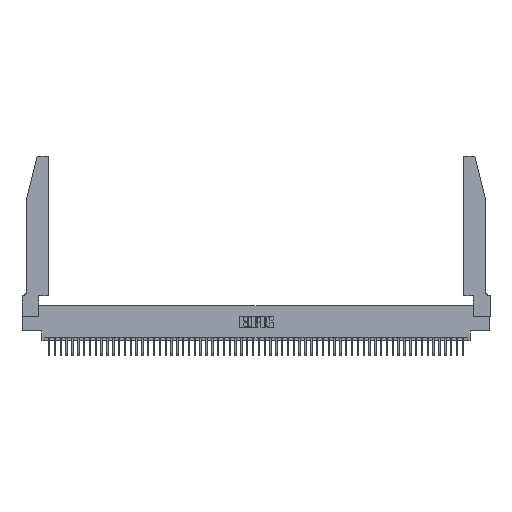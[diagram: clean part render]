
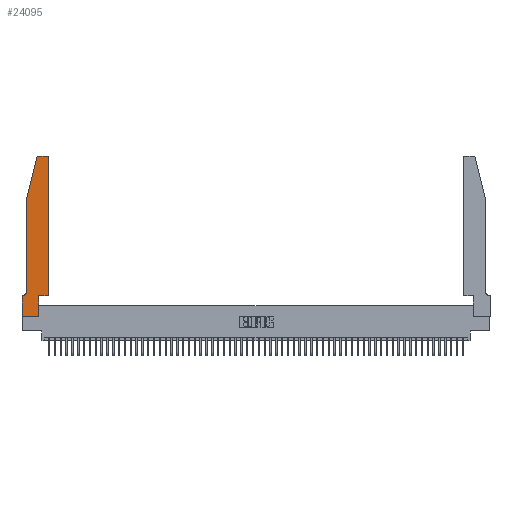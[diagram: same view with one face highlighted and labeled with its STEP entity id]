
A CAD part, top view. The second image highlights one B-rep face of the part: STEP entity #24095.
In plain terms, the highlighted planar face has unit normal (0, 0, 1).
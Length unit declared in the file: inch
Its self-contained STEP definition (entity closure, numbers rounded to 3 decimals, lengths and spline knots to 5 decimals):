
#337 = AXIS2_PLACEMENT_3D ( 'NONE', #19456, #49234, #23762 ) ;
#1120 = CARTESIAN_POINT ( 'NONE',  ( 0.4205, 2.75, 0.37 ) ) ;
#1465 = CARTESIAN_POINT ( 'NONE',  ( 0., 0., 0.37 ) ) ;
#1856 = AXIS2_PLACEMENT_3D ( 'NONE', #42576, #17095, #46843 ) ;
#1922 = AXIS2_PLACEMENT_3D ( 'NONE', #6892, #36635, #11171 ) ;
#1955 = EDGE_CURVE ( 'NONE', #13772, #27089, #21407, .T. ) ;
#2483 = AXIS2_PLACEMENT_3D ( 'NONE', #31450, #44285, #18793 ) ;
#2968 = DIRECTION ( 'NONE',  ( 0., -1., 0. ) ) ;
#3579 = CARTESIAN_POINT ( 'NONE',  ( 0., 0., 0.37 ) ) ;
#4374 = LINE ( 'NONE', #47335, #25653 ) ;
#4497 = CARTESIAN_POINT ( 'NONE',  ( 0.4505, 0.35, 0.37 ) ) ;
#4533 = LINE ( 'NONE', #18354, #25802 ) ;
#4956 = DIRECTION ( 'NONE',  ( 0., -1., 0. ) ) ;
#5201 = VECTOR ( 'NONE', #12156, 39.37008 ) ;
#5822 = CARTESIAN_POINT ( 'NONE',  ( 0.0755, 2., 0.37 ) ) ;
#6557 = LINE ( 'NONE', #3579, #5201 ) ;
#6892 = CARTESIAN_POINT ( 'NONE',  ( 0.0055, 0.42, 0.37 ) ) ;
#7888 = CIRCLE ( 'NONE', #337, 0.03 ) ;
#9234 = VERTEX_POINT ( 'NONE', #1120 ) ;
#11082 = VECTOR ( 'NONE', #4956, 39.37008 ) ;
#11171 = DIRECTION ( 'NONE',  ( -1., 0., 0. ) ) ;
#11307 = FACE_OUTER_BOUND ( 'NONE', #47465, .T. ) ;
#11352 = EDGE_CURVE ( 'NONE', #9234, #47479, #4374, .T. ) ;
#11476 = VECTOR ( 'NONE', #53965, 39.37008 ) ;
#11644 = CARTESIAN_POINT ( 'NONE',  ( 0.2865, 0.35, 0.37 ) ) ;
#11789 = VECTOR ( 'NONE', #41474, 39.37008 ) ;
#12156 = DIRECTION ( 'NONE',  ( 1., 0., 0. ) ) ;
#12590 = EDGE_CURVE ( 'NONE', #44897, #9234, #29508, .T. ) ;
#13052 = DIRECTION ( 'NONE',  ( 1., 0., 0. ) ) ;
#13772 = VERTEX_POINT ( 'NONE', #37748 ) ;
#14121 = EDGE_CURVE ( 'NONE', #33669, #23694, #28674, .T. ) ;
#15926 = ORIENTED_EDGE ( 'NONE', *, *, #1955, .T. ) ;
#16284 = EDGE_CURVE ( 'NONE', #50764, #33669, #6557, .T. ) ;
#17095 = DIRECTION ( 'NONE',  ( 0., 0., 1. ) ) ;
#17925 = CARTESIAN_POINT ( 'NONE',  ( 0., 0., 0.37 ) ) ;
#18354 = CARTESIAN_POINT ( 'NONE',  ( 0.4505, 0.35, 0.37 ) ) ;
#18793 = DIRECTION ( 'NONE',  ( 1., 0., 0. ) ) ;
#19456 = CARTESIAN_POINT ( 'NONE',  ( 0.284, 2.72, 0.37 ) ) ;
#21407 = LINE ( 'NONE', #37072, #11476 ) ;
#22044 = ORIENTED_EDGE ( 'NONE', *, *, #38626, .T. ) ;
#22248 = LINE ( 'NONE', #4497, #43533 ) ;
#23079 = LINE ( 'NONE', #37208, #11789 ) ;
#23194 = ORIENTED_EDGE ( 'NONE', *, *, #24812, .T. ) ;
#23694 = VERTEX_POINT ( 'NONE', #11644 ) ;
#23709 = LINE ( 'NONE', #17925, #11082 ) ;
#23762 = DIRECTION ( 'NONE',  ( 1., 0., 0. ) ) ;
#23833 = CARTESIAN_POINT ( 'NONE',  ( 0.4505, 0.35, 0.37 ) ) ;
#24095 = ADVANCED_FACE ( 'NONE', ( #11307 ), #40015, .T. ) ;
#24812 = EDGE_CURVE ( 'NONE', #47479, #26191, #7888, .T. ) ;
#25615 = EDGE_CURVE ( 'NONE', #26191, #43483, #23079, .T. ) ;
#25653 = VECTOR ( 'NONE', #43073, 39.37008 ) ;
#25802 = VECTOR ( 'NONE', #44057, 39.37008 ) ;
#26191 = VERTEX_POINT ( 'NONE', #28221 ) ;
#26787 = VERTEX_POINT ( 'NONE', #41174 ) ;
#27089 = VERTEX_POINT ( 'NONE', #39281 ) ;
#27273 = ORIENTED_EDGE ( 'NONE', *, *, #16284, .T. ) ;
#28084 = ORIENTED_EDGE ( 'NONE', *, *, #36572, .T. ) ;
#28221 = CARTESIAN_POINT ( 'NONE',  ( 0.25487, 2.72718, 0.37 ) ) ;
#28674 = LINE ( 'NONE', #31579, #41311 ) ;
#29508 = CIRCLE ( 'NONE', #1856, 0.03 ) ;
#30408 = CIRCLE ( 'NONE', #1922, 0.07 ) ;
#30502 = ORIENTED_EDGE ( 'NONE', *, *, #11352, .T. ) ;
#31216 = ORIENTED_EDGE ( 'NONE', *, *, #40775, .T. ) ;
#31450 = CARTESIAN_POINT ( 'NONE',  ( 0., 0.35, 0.37 ) ) ;
#31579 = CARTESIAN_POINT ( 'NONE',  ( 0.2865, 0.35, 0.37 ) ) ;
#31886 = ORIENTED_EDGE ( 'NONE', *, *, #25615, .T. ) ;
#32110 = VERTEX_POINT ( 'NONE', #23833 ) ;
#32732 = CARTESIAN_POINT ( 'NONE',  ( 0.0755, 2., 0.37 ) ) ;
#33669 = VERTEX_POINT ( 'NONE', #50611 ) ;
#35872 = DIRECTION ( 'NONE',  ( 0., 1., 0. ) ) ;
#36572 = EDGE_CURVE ( 'NONE', #32110, #44897, #4533, .T. ) ;
#36635 = DIRECTION ( 'NONE',  ( 0., 0., -1. ) ) ;
#36973 = CARTESIAN_POINT ( 'NONE',  ( 0.284, 2.75, 0.37 ) ) ;
#37072 = CARTESIAN_POINT ( 'NONE',  ( 0.0755, 0.35, 0.37 ) ) ;
#37187 = EDGE_CURVE ( 'NONE', #26787, #13772, #30408, .T. ) ;
#37208 = CARTESIAN_POINT ( 'NONE',  ( 0.0755, 2., 0.37 ) ) ;
#37517 = VECTOR ( 'NONE', #2968, 39.37008 ) ;
#37748 = CARTESIAN_POINT ( 'NONE',  ( 0.0055, 0.35, 0.37 ) ) ;
#38626 = EDGE_CURVE ( 'NONE', #23694, #32110, #22248, .T. ) ;
#38958 = EDGE_CURVE ( 'NONE', #43483, #26787, #50160, .T. ) ;
#39281 = CARTESIAN_POINT ( 'NONE',  ( 0., 0.35, 0.37 ) ) ;
#40015 = PLANE ( 'NONE',  #2483 ) ;
#40775 = EDGE_CURVE ( 'NONE', #27089, #50764, #23709, .T. ) ;
#41174 = CARTESIAN_POINT ( 'NONE',  ( 0.0755, 0.42, 0.37 ) ) ;
#41311 = VECTOR ( 'NONE', #35872, 39.37008 ) ;
#41474 = DIRECTION ( 'NONE',  ( -0.239, -0.971, 0. ) ) ;
#42576 = CARTESIAN_POINT ( 'NONE',  ( 0.4205, 2.72, 0.37 ) ) ;
#43073 = DIRECTION ( 'NONE',  ( -1., 0., 0. ) ) ;
#43483 = VERTEX_POINT ( 'NONE', #5822 ) ;
#43533 = VECTOR ( 'NONE', #13052, 39.37008 ) ;
#44057 = DIRECTION ( 'NONE',  ( 0., 1., 0. ) ) ;
#44285 = DIRECTION ( 'NONE',  ( 0., 0., 1. ) ) ;
#44897 = VERTEX_POINT ( 'NONE', #54198 ) ;
#46729 = ORIENTED_EDGE ( 'NONE', *, *, #12590, .T. ) ;
#46843 = DIRECTION ( 'NONE',  ( 1., 0., 0. ) ) ;
#47263 = ORIENTED_EDGE ( 'NONE', *, *, #14121, .T. ) ;
#47335 = CARTESIAN_POINT ( 'NONE',  ( 0.2605, 2.75, 0.37 ) ) ;
#47465 = EDGE_LOOP ( 'NONE', ( #30502, #23194, #31886, #47915, #52448, #15926, #31216, #27273, #47263, #22044, #28084, #46729 ) ) ;
#47479 = VERTEX_POINT ( 'NONE', #36973 ) ;
#47915 = ORIENTED_EDGE ( 'NONE', *, *, #38958, .T. ) ;
#49234 = DIRECTION ( 'NONE',  ( 0., 0., 1. ) ) ;
#50160 = LINE ( 'NONE', #32732, #37517 ) ;
#50611 = CARTESIAN_POINT ( 'NONE',  ( 0.2865, 0., 0.37 ) ) ;
#50764 = VERTEX_POINT ( 'NONE', #1465 ) ;
#52448 = ORIENTED_EDGE ( 'NONE', *, *, #37187, .T. ) ;
#53965 = DIRECTION ( 'NONE',  ( -1., 0., 0. ) ) ;
#54198 = CARTESIAN_POINT ( 'NONE',  ( 0.4505, 2.72, 0.37 ) ) ;
